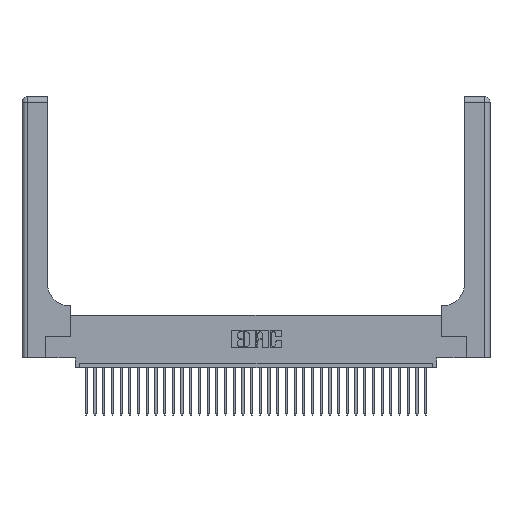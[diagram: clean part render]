
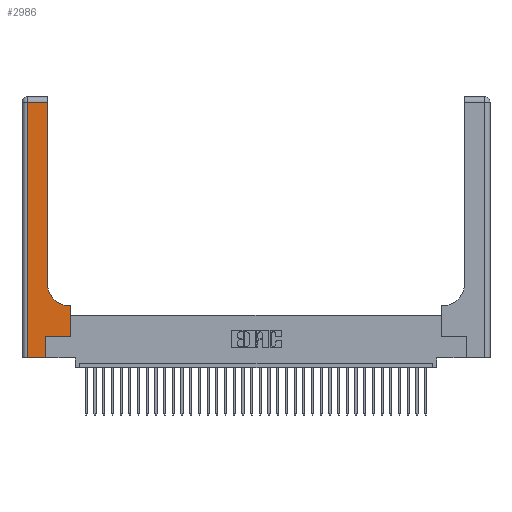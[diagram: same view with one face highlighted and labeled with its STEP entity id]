
A CAD part, top view. The second image highlights one B-rep face of the part: STEP entity #2986.
In plain terms, the highlighted planar face has unit normal (0, 0, 1).
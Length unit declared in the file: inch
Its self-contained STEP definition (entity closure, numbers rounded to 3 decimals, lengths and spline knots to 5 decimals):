
#623 = CIRCLE ( 'NONE', #14238, 0.25 ) ;
#1263 = PLANE ( 'NONE',  #25875 ) ;
#1516 = DIRECTION ( 'NONE',  ( -1., 0., 0. ) ) ;
#2016 = CARTESIAN_POINT ( 'NONE',  ( 0.06, 2.94, 0.37 ) ) ;
#2331 = EDGE_CURVE ( 'NONE', #6879, #21933, #22851, .T. ) ;
#2986 = ADVANCED_FACE ( 'NONE', ( #28407 ), #1263, .F. ) ;
#3414 = DIRECTION ( 'NONE',  ( 0., 1., 0. ) ) ;
#3843 = EDGE_CURVE ( 'NONE', #11767, #6879, #19696, .T. ) ;
#5532 = ORIENTED_EDGE ( 'NONE', *, *, #2331, .T. ) ;
#6464 = EDGE_CURVE ( 'NONE', #23652, #23547, #33056, .T. ) ;
#6779 = VECTOR ( 'NONE', #16929, 39.37008 ) ;
#6879 = VERTEX_POINT ( 'NONE', #8758 ) ;
#7216 = CARTESIAN_POINT ( 'NONE',  ( 0.269, 0., 0.37 ) ) ;
#8403 = VERTEX_POINT ( 'NONE', #22617 ) ;
#8414 = DIRECTION ( 'NONE',  ( -1., 0., 0. ) ) ;
#8758 = CARTESIAN_POINT ( 'NONE',  ( 0.5585, 0.6, 0.37 ) ) ;
#9712 = CARTESIAN_POINT ( 'NONE',  ( 0., 3., 0.37 ) ) ;
#9825 = DIRECTION ( 'NONE',  ( 1., 0., 0. ) ) ;
#9973 = CARTESIAN_POINT ( 'NONE',  ( 0.2915, 0.85, 0.37 ) ) ;
#11543 = ORIENTED_EDGE ( 'NONE', *, *, #21648, .T. ) ;
#11767 = VERTEX_POINT ( 'NONE', #19943 ) ;
#12162 = LINE ( 'NONE', #12934, #13084 ) ;
#12351 = VECTOR ( 'NONE', #34041, 39.37008 ) ;
#12934 = CARTESIAN_POINT ( 'NONE',  ( 0.2915, 3., 0.37 ) ) ;
#13016 = EDGE_CURVE ( 'NONE', #22133, #28319, #12162, .T. ) ;
#13084 = VECTOR ( 'NONE', #15958, 39.37008 ) ;
#13178 = CARTESIAN_POINT ( 'NONE',  ( 0.06, 3., 0.37 ) ) ;
#13492 = CARTESIAN_POINT ( 'NONE',  ( 0.269, 0.25, 0.37 ) ) ;
#13993 = ORIENTED_EDGE ( 'NONE', *, *, #18203, .T. ) ;
#14238 = AXIS2_PLACEMENT_3D ( 'NONE', #15399, #29028, #9825 ) ;
#14359 = ORIENTED_EDGE ( 'NONE', *, *, #13016, .T. ) ;
#14605 = VECTOR ( 'NONE', #17423, 39.37008 ) ;
#14799 = CARTESIAN_POINT ( 'NONE',  ( 0.2915, 2.94, 0.37 ) ) ;
#14864 = LINE ( 'NONE', #13178, #31241 ) ;
#15378 = EDGE_CURVE ( 'NONE', #23547, #8403, #22077, .T. ) ;
#15399 = CARTESIAN_POINT ( 'NONE',  ( 0.5415, 0.85, 0.37 ) ) ;
#15958 = DIRECTION ( 'NONE',  ( 0., 1., 0. ) ) ;
#16929 = DIRECTION ( 'NONE',  ( 1., 0., 0. ) ) ;
#17157 = ORIENTED_EDGE ( 'NONE', *, *, #15378, .T. ) ;
#17289 = CARTESIAN_POINT ( 'NONE',  ( 0., 0., 0.37 ) ) ;
#17390 = ORIENTED_EDGE ( 'NONE', *, *, #32480, .T. ) ;
#17423 = DIRECTION ( 'NONE',  ( -1., 0., 0. ) ) ;
#17669 = ORIENTED_EDGE ( 'NONE', *, *, #27823, .T. ) ;
#18066 = DIRECTION ( 'NONE',  ( 0., 0., -1. ) ) ;
#18203 = EDGE_CURVE ( 'NONE', #21933, #22133, #623, .T. ) ;
#19696 = LINE ( 'NONE', #20359, #12351 ) ;
#19943 = CARTESIAN_POINT ( 'NONE',  ( 0.5585, 0.25, 0.37 ) ) ;
#20359 = CARTESIAN_POINT ( 'NONE',  ( 0.5585, 0.25, 0.37 ) ) ;
#21643 = VECTOR ( 'NONE', #3414, 39.37008 ) ;
#21648 = EDGE_CURVE ( 'NONE', #28319, #33134, #31474, .T. ) ;
#21933 = VERTEX_POINT ( 'NONE', #30932 ) ;
#22077 = LINE ( 'NONE', #30003, #21643 ) ;
#22133 = VERTEX_POINT ( 'NONE', #9973 ) ;
#22617 = CARTESIAN_POINT ( 'NONE',  ( 0.269, 0.25, 0.37 ) ) ;
#22851 = LINE ( 'NONE', #25670, #14605 ) ;
#23547 = VERTEX_POINT ( 'NONE', #7216 ) ;
#23652 = VERTEX_POINT ( 'NONE', #31647 ) ;
#24307 = CARTESIAN_POINT ( 'NONE',  ( 0., 2.94, 0.37 ) ) ;
#24388 = ORIENTED_EDGE ( 'NONE', *, *, #6464, .T. ) ;
#24851 = LINE ( 'NONE', #13492, #30817 ) ;
#25670 = CARTESIAN_POINT ( 'NONE',  ( 0.2915, 0.6, 0.37 ) ) ;
#25875 = AXIS2_PLACEMENT_3D ( 'NONE', #9712, #18066, #1516 ) ;
#26500 = EDGE_LOOP ( 'NONE', ( #14359, #11543, #17390, #24388, #17157, #17669, #29937, #5532, #13993 ) ) ;
#26823 = VECTOR ( 'NONE', #8414, 39.37008 ) ;
#27302 = DIRECTION ( 'NONE',  ( 0., -1., 0. ) ) ;
#27823 = EDGE_CURVE ( 'NONE', #8403, #11767, #24851, .T. ) ;
#28319 = VERTEX_POINT ( 'NONE', #14799 ) ;
#28407 = FACE_OUTER_BOUND ( 'NONE', #26500, .T. ) ;
#29028 = DIRECTION ( 'NONE',  ( 0., 0., -1. ) ) ;
#29937 = ORIENTED_EDGE ( 'NONE', *, *, #3843, .T. ) ;
#30003 = CARTESIAN_POINT ( 'NONE',  ( 0.269, 0., 0.37 ) ) ;
#30800 = DIRECTION ( 'NONE',  ( 1., 0., 0. ) ) ;
#30817 = VECTOR ( 'NONE', #30800, 39.37008 ) ;
#30932 = CARTESIAN_POINT ( 'NONE',  ( 0.5415, 0.6, 0.37 ) ) ;
#31241 = VECTOR ( 'NONE', #27302, 39.37008 ) ;
#31474 = LINE ( 'NONE', #24307, #26823 ) ;
#31647 = CARTESIAN_POINT ( 'NONE',  ( 0.06, 0., 0.37 ) ) ;
#32480 = EDGE_CURVE ( 'NONE', #33134, #23652, #14864, .T. ) ;
#33056 = LINE ( 'NONE', #17289, #6779 ) ;
#33134 = VERTEX_POINT ( 'NONE', #2016 ) ;
#34041 = DIRECTION ( 'NONE',  ( 0., 1., 0. ) ) ;
